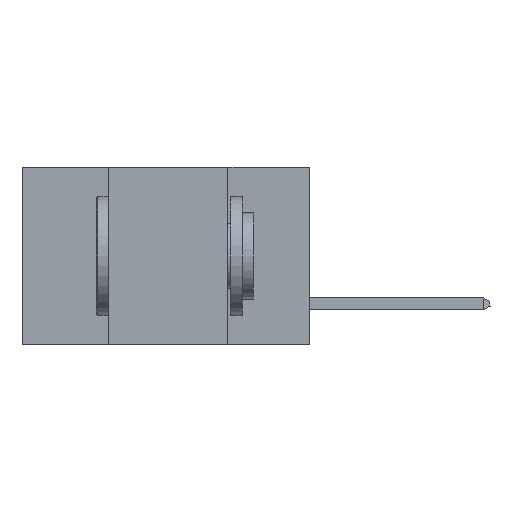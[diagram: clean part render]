
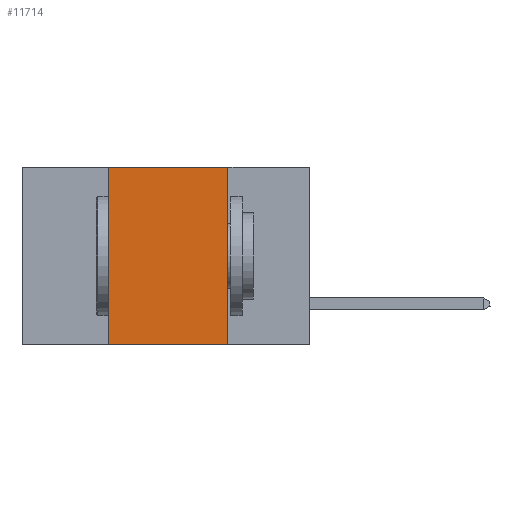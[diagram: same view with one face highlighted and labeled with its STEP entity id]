
A CAD part, left-side view. The second image highlights one B-rep face of the part: STEP entity #11714.
In plain terms, the highlighted planar face has unit normal (-1, 0, 0).
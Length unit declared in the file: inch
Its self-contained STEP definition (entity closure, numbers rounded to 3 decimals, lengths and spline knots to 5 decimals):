
#157 = CARTESIAN_POINT ( 'NONE',  ( 0., 0.17, 0. ) ) ;
#282 = DIRECTION ( 'NONE',  ( 0., 0., 1. ) ) ;
#725 = DIRECTION ( 'NONE',  ( 0., 0., -1. ) ) ;
#809 = VECTOR ( 'NONE', #8022, 39.37008 ) ;
#942 = DIRECTION ( 'NONE',  ( 0., -1., 0. ) ) ;
#3404 = VERTEX_POINT ( 'NONE', #157 ) ;
#4052 = LINE ( 'NONE', #32631, #809 ) ;
#4518 = DIRECTION ( 'NONE',  ( 0., -1., 0. ) ) ;
#4624 = ORIENTED_EDGE ( 'NONE', *, *, #38756, .F. ) ;
#4651 = ORIENTED_EDGE ( 'NONE', *, *, #24444, .T. ) ;
#4656 = PLANE ( 'NONE',  #22649 ) ;
#5021 = LINE ( 'NONE', #28089, #18121 ) ;
#6593 = VECTOR ( 'NONE', #4518, 39.37008 ) ;
#7707 = ORIENTED_EDGE ( 'NONE', *, *, #41790, .F. ) ;
#7735 = CARTESIAN_POINT ( 'NONE',  ( 0., 0.6, -0.37 ) ) ;
#8022 = DIRECTION ( 'NONE',  ( 0., 0., -1. ) ) ;
#11245 = CARTESIAN_POINT ( 'NONE',  ( 0., 0.6, 0. ) ) ;
#11714 = ADVANCED_FACE ( 'NONE', ( #20363 ), #4656, .F. ) ;
#17053 = VERTEX_POINT ( 'NONE', #32389 ) ;
#18121 = VECTOR ( 'NONE', #282, 39.37008 ) ;
#19482 = EDGE_LOOP ( 'NONE', ( #37797, #7707, #4624, #4651 ) ) ;
#20363 = FACE_OUTER_BOUND ( 'NONE', #19482, .T. ) ;
#22649 = AXIS2_PLACEMENT_3D ( 'NONE', #11245, #28998, #725 ) ;
#24444 = EDGE_CURVE ( 'NONE', #17053, #42944, #27948, .T. ) ;
#26909 = VECTOR ( 'NONE', #942, 39.37008 ) ;
#27948 = LINE ( 'NONE', #7735, #6593 ) ;
#28089 = CARTESIAN_POINT ( 'NONE',  ( 0., 0.42, 0. ) ) ;
#28417 = EDGE_CURVE ( 'NONE', #3404, #42944, #4052, .T. ) ;
#28998 = DIRECTION ( 'NONE',  ( 1., 0., 0. ) ) ;
#32389 = CARTESIAN_POINT ( 'NONE',  ( 0., 0.42, -0.37 ) ) ;
#32631 = CARTESIAN_POINT ( 'NONE',  ( 0., 0.17, 0. ) ) ;
#36072 = CARTESIAN_POINT ( 'NONE',  ( 0., 0.6, 0. ) ) ;
#37499 = CARTESIAN_POINT ( 'NONE',  ( 0., 0.42, 0. ) ) ;
#37797 = ORIENTED_EDGE ( 'NONE', *, *, #28417, .F. ) ;
#38756 = EDGE_CURVE ( 'NONE', #17053, #41332, #5021, .T. ) ;
#39648 = CARTESIAN_POINT ( 'NONE',  ( 0., 0.17, -0.37 ) ) ;
#41332 = VERTEX_POINT ( 'NONE', #37499 ) ;
#41790 = EDGE_CURVE ( 'NONE', #41332, #3404, #43953, .T. ) ;
#42944 = VERTEX_POINT ( 'NONE', #39648 ) ;
#43953 = LINE ( 'NONE', #36072, #26909 ) ;
